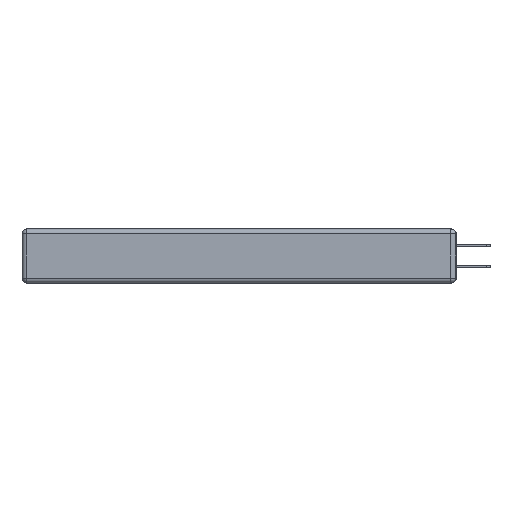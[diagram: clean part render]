
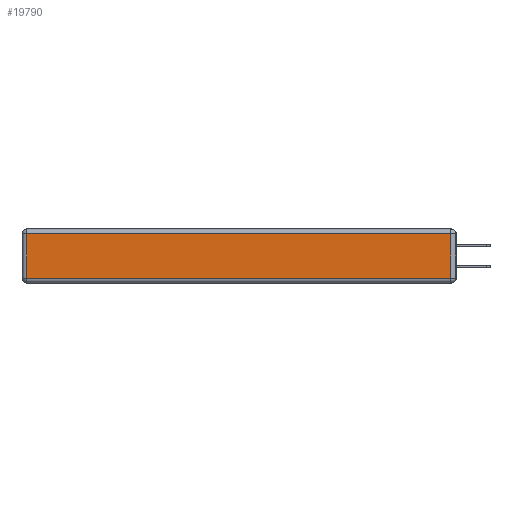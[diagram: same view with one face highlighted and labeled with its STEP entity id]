
A CAD part, left-side view. The second image highlights one B-rep face of the part: STEP entity #19790.
In plain terms, the highlighted planar face has unit normal (-1, 0, 0).
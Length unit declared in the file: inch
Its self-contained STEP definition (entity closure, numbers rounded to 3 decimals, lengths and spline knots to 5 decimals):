
#1081 = CARTESIAN_POINT ( 'NONE',  ( 0., 0.03, -0.313 ) ) ;
#2174 = DIRECTION ( 'NONE',  ( 0., 0., -1. ) ) ;
#2964 = DIRECTION ( 'NONE',  ( -1., 0., 0. ) ) ;
#3134 = VERTEX_POINT ( 'NONE', #9024 ) ;
#5428 = VERTEX_POINT ( 'NONE', #7994 ) ;
#5934 = CARTESIAN_POINT ( 'NONE',  ( 0., 0., -0.313 ) ) ;
#7599 = EDGE_CURVE ( 'NONE', #5428, #8781, #7990, .T. ) ;
#7990 = LINE ( 'NONE', #5934, #13387 ) ;
#7994 = CARTESIAN_POINT ( 'NONE',  ( 0., 2.72, -0.313 ) ) ;
#8343 = AXIS2_PLACEMENT_3D ( 'NONE', #9633, #2964, #14570 ) ;
#8517 = ORIENTED_EDGE ( 'NONE', *, *, #7599, .T. ) ;
#8637 = VECTOR ( 'NONE', #9975, 39.37008 ) ;
#8781 = VERTEX_POINT ( 'NONE', #1081 ) ;
#9024 = CARTESIAN_POINT ( 'NONE',  ( 0., 0.03, -0.03 ) ) ;
#9633 = CARTESIAN_POINT ( 'NONE',  ( 0., 0., -0.343 ) ) ;
#9975 = DIRECTION ( 'NONE',  ( 0., 0., 1. ) ) ;
#10140 = EDGE_CURVE ( 'NONE', #8781, #3134, #13017, .T. ) ;
#11090 = ORIENTED_EDGE ( 'NONE', *, *, #10140, .T. ) ;
#11985 = VERTEX_POINT ( 'NONE', #20120 ) ;
#12577 = DIRECTION ( 'NONE',  ( 0., -1., 0. ) ) ;
#13017 = LINE ( 'NONE', #14961, #8637 ) ;
#13279 = EDGE_CURVE ( 'NONE', #11985, #5428, #14784, .T. ) ;
#13387 = VECTOR ( 'NONE', #12577, 39.37008 ) ;
#13583 = EDGE_LOOP ( 'NONE', ( #8517, #11090, #19276, #16889 ) ) ;
#13636 = CARTESIAN_POINT ( 'NONE',  ( 0., 2.72, -0.343 ) ) ;
#14570 = DIRECTION ( 'NONE',  ( 0., 0., 1. ) ) ;
#14784 = LINE ( 'NONE', #13636, #20193 ) ;
#14961 = CARTESIAN_POINT ( 'NONE',  ( 0., 0.03, -0.343 ) ) ;
#16786 = EDGE_CURVE ( 'NONE', #3134, #11985, #20534, .T. ) ;
#16889 = ORIENTED_EDGE ( 'NONE', *, *, #13279, .T. ) ;
#16945 = FACE_OUTER_BOUND ( 'NONE', #13583, .T. ) ;
#18006 = CARTESIAN_POINT ( 'NONE',  ( 0., 2.75, -0.03 ) ) ;
#19276 = ORIENTED_EDGE ( 'NONE', *, *, #16786, .T. ) ;
#19448 = PLANE ( 'NONE',  #8343 ) ;
#19507 = VECTOR ( 'NONE', #21139, 39.37008 ) ;
#19790 = ADVANCED_FACE ( 'NONE', ( #16945 ), #19448, .T. ) ;
#20120 = CARTESIAN_POINT ( 'NONE',  ( 0., 2.72, -0.03 ) ) ;
#20193 = VECTOR ( 'NONE', #2174, 39.37008 ) ;
#20534 = LINE ( 'NONE', #18006, #19507 ) ;
#21139 = DIRECTION ( 'NONE',  ( 0., 1., 0. ) ) ;
